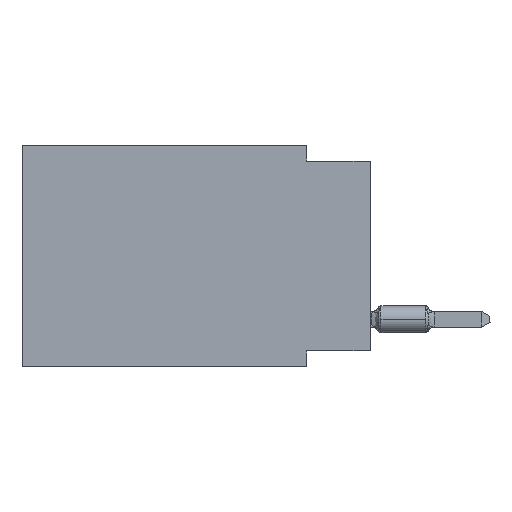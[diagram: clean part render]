
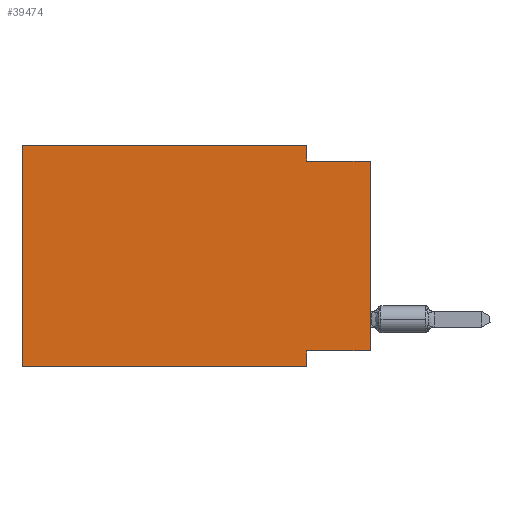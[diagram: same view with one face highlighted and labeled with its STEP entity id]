
A CAD part, left-side view. The second image highlights one B-rep face of the part: STEP entity #39474.
In plain terms, the highlighted planar face has unit normal (-1, 0, 0).
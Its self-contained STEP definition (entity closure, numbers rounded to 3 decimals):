
#1003 = ORIENTED_EDGE ( 'NONE', *, *, #23916, .F. ) ;
#1663 = LINE ( 'NONE', #17501, #39555 ) ;
#1765 = VERTEX_POINT ( 'NONE', #5022 ) ;
#2409 = LINE ( 'NONE', #40191, #34870 ) ;
#3271 = CARTESIAN_POINT ( 'NONE',  ( 0., 13.97, -8.89 ) ) ;
#4211 = VECTOR ( 'NONE', #16535, 1000. ) ;
#4381 = DIRECTION ( 'NONE',  ( 0., 1., 0. ) ) ;
#4919 = CARTESIAN_POINT ( 'NONE',  ( 0., 2.54, -8.89 ) ) ;
#5022 = CARTESIAN_POINT ( 'NONE',  ( 0., 2.54, 0. ) ) ;
#5611 = DIRECTION ( 'NONE',  ( 0., 0., -1. ) ) ;
#5743 = VERTEX_POINT ( 'NONE', #4919 ) ;
#6307 = CARTESIAN_POINT ( 'NONE',  ( 0., 13.97, 0. ) ) ;
#6886 = LINE ( 'NONE', #35477, #28640 ) ;
#6989 = CARTESIAN_POINT ( 'NONE',  ( 0., 2.54, 0. ) ) ;
#7769 = LINE ( 'NONE', #23415, #4211 ) ;
#8358 = ORIENTED_EDGE ( 'NONE', *, *, #13459, .F. ) ;
#8479 = VERTEX_POINT ( 'NONE', #13433 ) ;
#10538 = VERTEX_POINT ( 'NONE', #29958 ) ;
#11952 = AXIS2_PLACEMENT_3D ( 'NONE', #6307, #15470, #25490 ) ;
#11969 = VERTEX_POINT ( 'NONE', #31022 ) ;
#13137 = DIRECTION ( 'NONE',  ( 0., -1., 0. ) ) ;
#13433 = CARTESIAN_POINT ( 'NONE',  ( 0., 13.97, 0. ) ) ;
#13459 = EDGE_CURVE ( 'NONE', #34978, #8479, #7769, .T. ) ;
#13958 = EDGE_CURVE ( 'NONE', #10538, #5743, #1663, .T. ) ;
#14167 = LINE ( 'NONE', #29637, #38986 ) ;
#14832 = CARTESIAN_POINT ( 'NONE',  ( 0., 0., -0.635 ) ) ;
#15126 = ORIENTED_EDGE ( 'NONE', *, *, #40309, .T. ) ;
#15159 = DIRECTION ( 'NONE',  ( 0., -1., 0. ) ) ;
#15470 = DIRECTION ( 'NONE',  ( 1., 0., 0. ) ) ;
#16535 = DIRECTION ( 'NONE',  ( 0., 0., 1. ) ) ;
#17501 = CARTESIAN_POINT ( 'NONE',  ( 0., 2.54, -8.89 ) ) ;
#20469 = CARTESIAN_POINT ( 'NONE',  ( 0., 0., -0.635 ) ) ;
#23224 = CARTESIAN_POINT ( 'NONE',  ( 0., 2.54, -0.635 ) ) ;
#23351 = DIRECTION ( 'NONE',  ( 0., 0., 1. ) ) ;
#23415 = CARTESIAN_POINT ( 'NONE',  ( 0., 13.97, 0. ) ) ;
#23477 = VERTEX_POINT ( 'NONE', #20469 ) ;
#23916 = EDGE_CURVE ( 'NONE', #11969, #10538, #14167, .T. ) ;
#25490 = DIRECTION ( 'NONE',  ( 0., 0., -1. ) ) ;
#25690 = EDGE_CURVE ( 'NONE', #32762, #23477, #29874, .T. ) ;
#26373 = LINE ( 'NONE', #6989, #33917 ) ;
#26881 = EDGE_CURVE ( 'NONE', #11969, #23477, #2409, .T. ) ;
#27659 = ORIENTED_EDGE ( 'NONE', *, *, #13958, .F. ) ;
#27924 = EDGE_LOOP ( 'NONE', ( #36131, #40906, #34293, #38664, #8358, #15126, #27659, #1003 ) ) ;
#28640 = VECTOR ( 'NONE', #13137, 1000. ) ;
#29637 = CARTESIAN_POINT ( 'NONE',  ( 0., 0., -8.255 ) ) ;
#29874 = LINE ( 'NONE', #14832, #32750 ) ;
#29958 = CARTESIAN_POINT ( 'NONE',  ( 0., 2.54, -8.255 ) ) ;
#31022 = CARTESIAN_POINT ( 'NONE',  ( 0., 0., -8.255 ) ) ;
#31031 = CARTESIAN_POINT ( 'NONE',  ( 0., 13.97, 0. ) ) ;
#32750 = VECTOR ( 'NONE', #39884, 1000. ) ;
#32762 = VERTEX_POINT ( 'NONE', #23224 ) ;
#33917 = VECTOR ( 'NONE', #39115, 1000. ) ;
#34293 = ORIENTED_EDGE ( 'NONE', *, *, #39250, .F. ) ;
#34870 = VECTOR ( 'NONE', #23351, 1000. ) ;
#34902 = PLANE ( 'NONE',  #11952 ) ;
#34978 = VERTEX_POINT ( 'NONE', #3271 ) ;
#35477 = CARTESIAN_POINT ( 'NONE',  ( 0., 13.97, -8.89 ) ) ;
#36131 = ORIENTED_EDGE ( 'NONE', *, *, #26881, .T. ) ;
#38239 = FACE_OUTER_BOUND ( 'NONE', #27924, .T. ) ;
#38664 = ORIENTED_EDGE ( 'NONE', *, *, #39736, .F. ) ;
#38986 = VECTOR ( 'NONE', #4381, 1000. ) ;
#39115 = DIRECTION ( 'NONE',  ( 0., 0., -1. ) ) ;
#39250 = EDGE_CURVE ( 'NONE', #1765, #32762, #26373, .T. ) ;
#39332 = VECTOR ( 'NONE', #15159, 1000. ) ;
#39474 = ADVANCED_FACE ( 'NONE', ( #38239 ), #34902, .F. ) ;
#39555 = VECTOR ( 'NONE', #5611, 1000. ) ;
#39736 = EDGE_CURVE ( 'NONE', #8479, #1765, #40638, .T. ) ;
#39884 = DIRECTION ( 'NONE',  ( 0., -1., 0. ) ) ;
#40191 = CARTESIAN_POINT ( 'NONE',  ( 0., 0., 0. ) ) ;
#40309 = EDGE_CURVE ( 'NONE', #34978, #5743, #6886, .T. ) ;
#40638 = LINE ( 'NONE', #31031, #39332 ) ;
#40906 = ORIENTED_EDGE ( 'NONE', *, *, #25690, .F. ) ;
